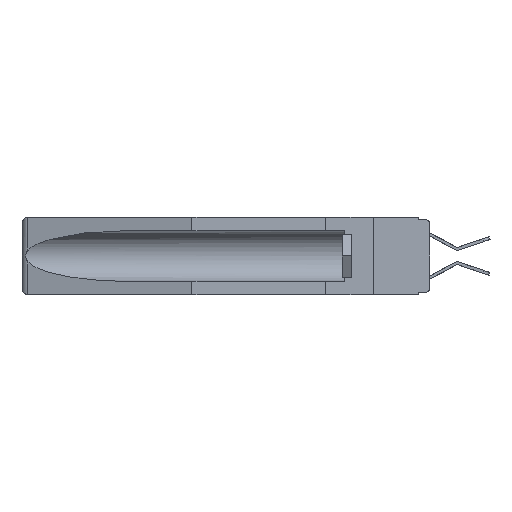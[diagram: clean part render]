
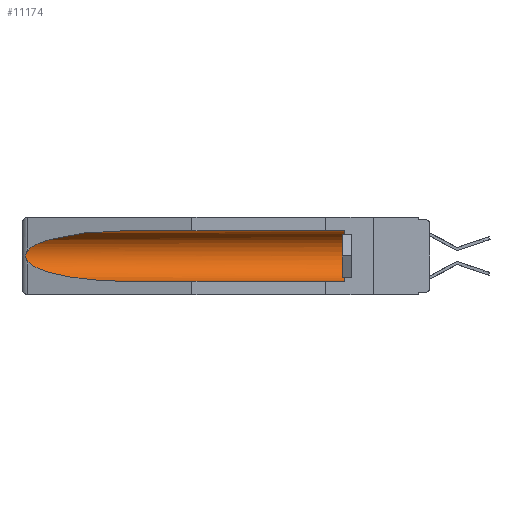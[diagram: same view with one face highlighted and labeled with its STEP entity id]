
A CAD part, left-side view. The second image highlights one B-rep face of the part: STEP entity #11174.
In plain terms, the highlighted cylindrical face has radius 2.857 mm (diameter 5.715 mm), a partial arc.
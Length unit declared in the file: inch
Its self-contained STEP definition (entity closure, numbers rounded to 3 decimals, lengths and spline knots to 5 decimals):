
#371 = CARTESIAN_POINT ( 'NONE',  ( 0.155, 1.07973, -0.284 ) ) ;
#620 = CARTESIAN_POINT ( 'NONE',  ( 0.155, 1.07973, -0.059 ) ) ;
#897 = EDGE_CURVE ( 'NONE', #10366, #14876, #22155, .T. ) ;
#1033 = CARTESIAN_POINT ( 'NONE',  ( 0.2673, 1.5327, -0.16383 ) ) ;
#2158 = ORIENTED_EDGE ( 'NONE', *, *, #7425, .F. ) ;
#2421 = LINE ( 'NONE', #20405, #23242 ) ;
#2578 = ORIENTED_EDGE ( 'NONE', *, *, #11764, .T. ) ;
#2598 = CARTESIAN_POINT ( 'NONE',  ( 0.26537, 1.52718, -0.14972 ) ) ;
#2784 = CARTESIAN_POINT ( 'NONE',  ( 0.155, -0.30754, -0.1715 ) ) ;
#3502 = VERTEX_POINT ( 'NONE', #18203 ) ;
#3824 = DIRECTION ( 'NONE',  ( 0., 1., 0. ) ) ;
#3934 = CARTESIAN_POINT ( 'NONE',  ( 0.21114, 1.30732, -0.284 ) ) ;
#5087 = FACE_OUTER_BOUND ( 'NONE', #17775, .T. ) ;
#6751 = VERTEX_POINT ( 'NONE', #11810 ) ;
#6774 = ORIENTED_EDGE ( 'NONE', *, *, #14632, .T. ) ;
#7154 = CARTESIAN_POINT ( 'NONE',  ( 0.26537, 1.52718, -0.14972 ) ) ;
#7425 = EDGE_CURVE ( 'NONE', #6751, #15973, #2421, .T. ) ;
#7428 = CARTESIAN_POINT ( 'NONE',  ( 0.26654, 1.53092, -0.15636 ) ) ;
#7956 = B_SPLINE_CURVE_WITH_KNOTS ( 'NONE', 3,
 ( #7154, #22087, #7428, #1033, #9469, #9273, #15602, #9371, #24104, #24188 ),
 .UNSPECIFIED., .F., .F.,
 ( 4, 2, 2, 2, 4 ),
 ( 0., 0.00029, 0.00058, 0.00087, 0.00117 ),
 .UNSPECIFIED. ) ;
#8467 = AXIS2_PLACEMENT_3D ( 'NONE', #2784, #8921, #11038 ) ;
#8509 = CARTESIAN_POINT ( 'NONE',  ( 0.155, 0.126, -0.1715 ) ) ;
#8633 = VECTOR ( 'NONE', #3824, 39.37008 ) ;
#8921 = DIRECTION ( 'NONE',  ( 0., 1., 0. ) ) ;
#9181 = CARTESIAN_POINT ( 'NONE',  ( 0.155, 1.07973, -0.059 ) ) ;
#9273 = CARTESIAN_POINT ( 'NONE',  ( 0.2675, 1.53308, -0.17534 ) ) ;
#9371 = CARTESIAN_POINT ( 'NONE',  ( 0.26655, 1.53094, -0.18657 ) ) ;
#9469 = CARTESIAN_POINT ( 'NONE',  ( 0.2675, 1.53308, -0.16763 ) ) ;
#10115 = CARTESIAN_POINT ( 'NONE',  ( 0.155, -0.30754, -0.059 ) ) ;
#10366 = VERTEX_POINT ( 'NONE', #10974 ) ;
#10974 = CARTESIAN_POINT ( 'NONE',  ( 0.155, 0.126, -0.059 ) ) ;
#11038 = DIRECTION ( 'NONE',  ( 0., 0., 1. ) ) ;
#11174 = ADVANCED_FACE ( 'NONE', ( #5087 ), #18624, .F. ) ;
#11671 =( BOUNDED_CURVE ( )  B_SPLINE_CURVE ( 3, ( #9181, #17451, #19490, #2598 ),
 .UNSPECIFIED., .F., .F. ) 
 B_SPLINE_CURVE_WITH_KNOTS ( ( 4, 4 ),
 ( 4.71239, 6.08839 ),
 .UNSPECIFIED. ) 
 CURVE ( )  GEOMETRIC_REPRESENTATION_ITEM ( )  RATIONAL_B_SPLINE_CURVE ( ( 1., 0.848, 0.848, 1. ) ) 
 REPRESENTATION_ITEM ( '' )  );
#11764 = EDGE_CURVE ( 'NONE', #3502, #15973, #16535, .T. ) ;
#11810 = CARTESIAN_POINT ( 'NONE',  ( 0.155, 0.126, -0.284 ) ) ;
#12045 = CARTESIAN_POINT ( 'NONE',  ( 0.25451, 1.48313, -0.24835 ) ) ;
#12831 = DIRECTION ( 'NONE',  ( 0., 0., 1. ) ) ;
#14632 = EDGE_CURVE ( 'NONE', #14876, #20446, #11671, .T. ) ;
#14783 = EDGE_CURVE ( 'NONE', #20446, #3502, #7956, .T. ) ;
#14876 = VERTEX_POINT ( 'NONE', #620 ) ;
#15297 = CIRCLE ( 'NONE', #15756, 0.1125 ) ;
#15602 = CARTESIAN_POINT ( 'NONE',  ( 0.2673, 1.53269, -0.17917 ) ) ;
#15756 = AXIS2_PLACEMENT_3D ( 'NONE', #8509, #25373, #12831 ) ;
#15973 = VERTEX_POINT ( 'NONE', #21039 ) ;
#16535 =( BOUNDED_CURVE ( )  B_SPLINE_CURVE ( 3, ( #25024, #12045, #3934, #371 ),
 .UNSPECIFIED., .F., .T. ) 
 B_SPLINE_CURVE_WITH_KNOTS ( ( 4, 4 ),
 ( 0.1948, 1.5708 ),
 .UNSPECIFIED. ) 
 CURVE ( )  GEOMETRIC_REPRESENTATION_ITEM ( )  RATIONAL_B_SPLINE_CURVE ( ( 1., 0.848, 0.848, 1. ) ) 
 REPRESENTATION_ITEM ( '' )  );
#17451 = CARTESIAN_POINT ( 'NONE',  ( 0.21114, 1.30732, -0.059 ) ) ;
#17510 = ORIENTED_EDGE ( 'NONE', *, *, #14783, .T. ) ;
#17775 = EDGE_LOOP ( 'NONE', ( #6774, #17510, #2578, #2158, #24632, #20192 ) ) ;
#18203 = CARTESIAN_POINT ( 'NONE',  ( 0.26537, 1.52718, -0.19328 ) ) ;
#18236 = CARTESIAN_POINT ( 'NONE',  ( 0.26537, 1.52718, -0.14972 ) ) ;
#18624 = CYLINDRICAL_SURFACE ( 'NONE', #8467, 0.1125 ) ;
#19490 = CARTESIAN_POINT ( 'NONE',  ( 0.25451, 1.48313, -0.09465 ) ) ;
#20192 = ORIENTED_EDGE ( 'NONE', *, *, #897, .T. ) ;
#20405 = CARTESIAN_POINT ( 'NONE',  ( 0.155, -0.30754, -0.284 ) ) ;
#20446 = VERTEX_POINT ( 'NONE', #18236 ) ;
#21039 = CARTESIAN_POINT ( 'NONE',  ( 0.155, 1.07973, -0.284 ) ) ;
#22087 = CARTESIAN_POINT ( 'NONE',  ( 0.26597, 1.52961, -0.15275 ) ) ;
#22155 = LINE ( 'NONE', #10115, #8633 ) ;
#22636 = DIRECTION ( 'NONE',  ( 0., 1., 0. ) ) ;
#23242 = VECTOR ( 'NONE', #22636, 39.37008 ) ;
#24104 = CARTESIAN_POINT ( 'NONE',  ( 0.26597, 1.5296, -0.19026 ) ) ;
#24188 = CARTESIAN_POINT ( 'NONE',  ( 0.26537, 1.52718, -0.19328 ) ) ;
#24632 = ORIENTED_EDGE ( 'NONE', *, *, #25399, .T. ) ;
#25024 = CARTESIAN_POINT ( 'NONE',  ( 0.26537, 1.52718, -0.19328 ) ) ;
#25373 = DIRECTION ( 'NONE',  ( 0., -1., 0. ) ) ;
#25399 = EDGE_CURVE ( 'NONE', #6751, #10366, #15297, .T. ) ;
